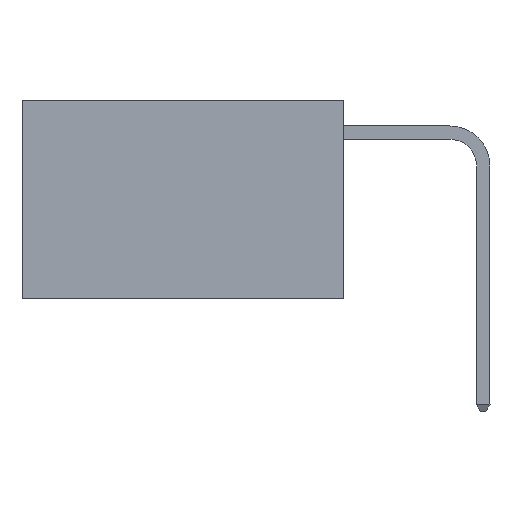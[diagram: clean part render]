
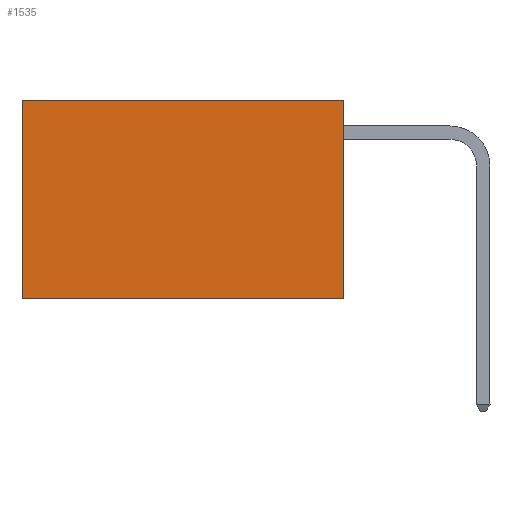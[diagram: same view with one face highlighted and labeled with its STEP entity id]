
A CAD part, left-side view. The second image highlights one B-rep face of the part: STEP entity #1535.
In plain terms, the highlighted planar face has unit normal (-1, 0, 0).
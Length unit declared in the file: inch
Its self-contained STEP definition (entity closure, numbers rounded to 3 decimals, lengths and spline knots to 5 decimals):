
#34 = ORIENTED_EDGE ( 'NONE', *, *, #7300, .F. ) ;
#39 = CARTESIAN_POINT ( 'NONE',  ( 0.2625, 0., 0. ) ) ;
#216 = VECTOR ( 'NONE', #1406, 39.37008 ) ;
#229 = EDGE_LOOP ( 'NONE', ( #7765, #34, #540, #323 ) ) ;
#323 = ORIENTED_EDGE ( 'NONE', *, *, #5357, .T. ) ;
#406 = CARTESIAN_POINT ( 'NONE',  ( 0.2625, 0., 0. ) ) ;
#481 = DIRECTION ( 'NONE',  ( 0., 0., -1. ) ) ;
#540 = ORIENTED_EDGE ( 'NONE', *, *, #2437, .F. ) ;
#562 = VERTEX_POINT ( 'NONE', #956 ) ;
#575 = FACE_OUTER_BOUND ( 'NONE', #229, .T. ) ;
#737 = CARTESIAN_POINT ( 'NONE',  ( 0.2625, 0.6, 0. ) ) ;
#956 = CARTESIAN_POINT ( 'NONE',  ( 0.2625, 0., -0.37 ) ) ;
#1406 = DIRECTION ( 'NONE',  ( 0., 0., -1. ) ) ;
#1535 = ADVANCED_FACE ( 'NONE', ( #575 ), #2276, .F. ) ;
#1801 = CARTESIAN_POINT ( 'NONE',  ( 0.2625, 0.6, 0. ) ) ;
#2026 = VECTOR ( 'NONE', #481, 39.37008 ) ;
#2241 = LINE ( 'NONE', #39, #2026 ) ;
#2266 = CARTESIAN_POINT ( 'NONE',  ( 0.2625, 0., 0. ) ) ;
#2276 = PLANE ( 'NONE',  #7759 ) ;
#2294 = DIRECTION ( 'NONE',  ( 0., 1., 0. ) ) ;
#2362 = DIRECTION ( 'NONE',  ( 0., 0., -1. ) ) ;
#2428 = LINE ( 'NONE', #737, #216 ) ;
#2437 = EDGE_CURVE ( 'NONE', #5931, #562, #2241, .T. ) ;
#3322 = VECTOR ( 'NONE', #3539, 39.37008 ) ;
#3539 = DIRECTION ( 'NONE',  ( 0., 1., 0. ) ) ;
#3623 = VERTEX_POINT ( 'NONE', #5485 ) ;
#4016 = VERTEX_POINT ( 'NONE', #1801 ) ;
#4171 = CARTESIAN_POINT ( 'NONE',  ( 0.2625, 0., -0.37 ) ) ;
#4297 = DIRECTION ( 'NONE',  ( 1., 0., 0. ) ) ;
#4987 = LINE ( 'NONE', #4171, #3322 ) ;
#5331 = VECTOR ( 'NONE', #2294, 39.37008 ) ;
#5357 = EDGE_CURVE ( 'NONE', #5931, #4016, #6760, .T. ) ;
#5376 = CARTESIAN_POINT ( 'NONE',  ( 0.2625, 0., 0. ) ) ;
#5485 = CARTESIAN_POINT ( 'NONE',  ( 0.2625, 0.6, -0.37 ) ) ;
#5931 = VERTEX_POINT ( 'NONE', #5376 ) ;
#6760 = LINE ( 'NONE', #2266, #5331 ) ;
#7300 = EDGE_CURVE ( 'NONE', #562, #3623, #4987, .T. ) ;
#7759 = AXIS2_PLACEMENT_3D ( 'NONE', #406, #4297, #2362 ) ;
#7765 = ORIENTED_EDGE ( 'NONE', *, *, #8018, .T. ) ;
#8018 = EDGE_CURVE ( 'NONE', #4016, #3623, #2428, .T. ) ;
